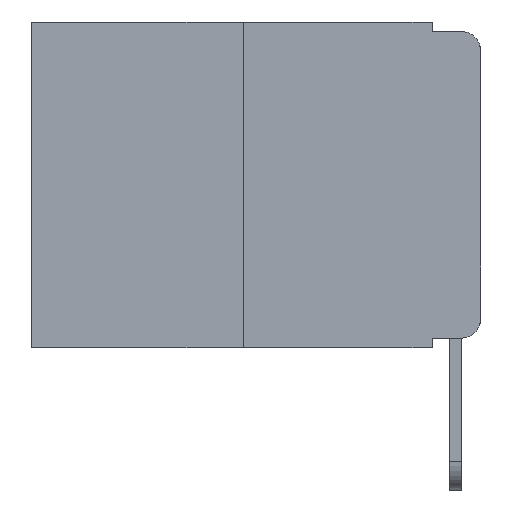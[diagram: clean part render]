
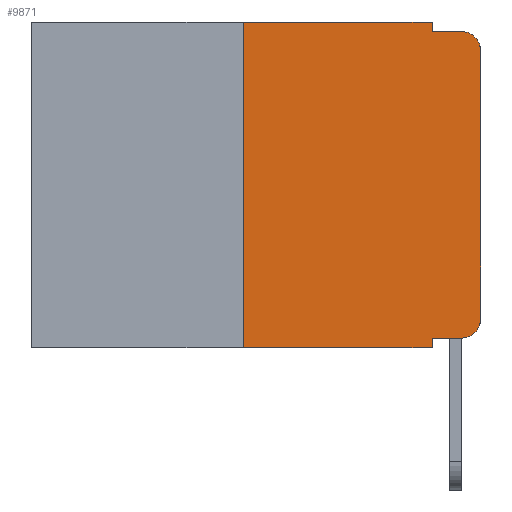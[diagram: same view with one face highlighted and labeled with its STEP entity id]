
A CAD part, left-side view. The second image highlights one B-rep face of the part: STEP entity #9871.
In plain terms, the highlighted planar face has unit normal (-1, 0, 0).
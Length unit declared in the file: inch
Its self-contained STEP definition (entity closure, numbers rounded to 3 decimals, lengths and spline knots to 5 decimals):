
#379 = DIRECTION ( 'NONE',  ( 0., 0., -1. ) ) ;
#418 = VECTOR ( 'NONE', #8810, 39.37008 ) ;
#495 = DIRECTION ( 'NONE',  ( 0., 0., -1. ) ) ;
#585 = ORIENTED_EDGE ( 'NONE', *, *, #9537, .T. ) ;
#765 = CARTESIAN_POINT ( 'NONE',  ( 0., 0.473, 0. ) ) ;
#1775 = CARTESIAN_POINT ( 'NONE',  ( 0., 0.473, 0. ) ) ;
#1841 = EDGE_CURVE ( 'NONE', #3556, #6633, #4339, .T. ) ;
#2386 = AXIS2_PLACEMENT_3D ( 'NONE', #2842, #4954, #379 ) ;
#2530 = VERTEX_POINT ( 'NONE', #12695 ) ;
#2642 = ORIENTED_EDGE ( 'NONE', *, *, #1841, .T. ) ;
#2717 = EDGE_LOOP ( 'NONE', ( #585, #4007, #13675, #11287, #14692, #12070, #2642, #13159, #13503, #4212 ) ) ;
#2809 = VERTEX_POINT ( 'NONE', #5738 ) ;
#2842 = CARTESIAN_POINT ( 'NONE',  ( 0., 0.02, -0.313 ) ) ;
#3222 = VERTEX_POINT ( 'NONE', #5618 ) ;
#3536 = DIRECTION ( 'NONE',  ( 0., -1., 0. ) ) ;
#3556 = VERTEX_POINT ( 'NONE', #5832 ) ;
#3585 = VECTOR ( 'NONE', #3536, 39.37008 ) ;
#3656 = VECTOR ( 'NONE', #9471, 39.37008 ) ;
#4007 = ORIENTED_EDGE ( 'NONE', *, *, #11040, .T. ) ;
#4096 = CARTESIAN_POINT ( 'NONE',  ( 0., 0., -0.03 ) ) ;
#4164 = LINE ( 'NONE', #7199, #13109 ) ;
#4197 = EDGE_CURVE ( 'NONE', #3222, #6633, #5877, .T. ) ;
#4212 = ORIENTED_EDGE ( 'NONE', *, *, #8658, .T. ) ;
#4235 = VERTEX_POINT ( 'NONE', #12694 ) ;
#4339 = LINE ( 'NONE', #8033, #3585 ) ;
#4785 = CARTESIAN_POINT ( 'NONE',  ( 0., 0.051, 0. ) ) ;
#4954 = DIRECTION ( 'NONE',  ( -1., 0., 0. ) ) ;
#5037 = LINE ( 'NONE', #11932, #14226 ) ;
#5238 = VECTOR ( 'NONE', #8023, 39.37008 ) ;
#5289 = CARTESIAN_POINT ( 'NONE',  ( 0., 0.051, 0. ) ) ;
#5618 = CARTESIAN_POINT ( 'NONE',  ( 0., 0.051, -0.333 ) ) ;
#5738 = CARTESIAN_POINT ( 'NONE',  ( 0., 0.051, 0. ) ) ;
#5832 = CARTESIAN_POINT ( 'NONE',  ( 0., 0.25, -0.343 ) ) ;
#5877 = LINE ( 'NONE', #4785, #11967 ) ;
#5885 = EDGE_CURVE ( 'NONE', #3556, #14198, #10777, .T. ) ;
#6035 = DIRECTION ( 'NONE',  ( -1., 0., 0. ) ) ;
#6120 = VERTEX_POINT ( 'NONE', #12020 ) ;
#6210 = LINE ( 'NONE', #765, #3656 ) ;
#6511 = DIRECTION ( 'NONE',  ( 0., 0., -1. ) ) ;
#6549 = VERTEX_POINT ( 'NONE', #14312 ) ;
#6633 = VERTEX_POINT ( 'NONE', #14507 ) ;
#7199 = CARTESIAN_POINT ( 'NONE',  ( 0., 0.051, -0.333 ) ) ;
#8023 = DIRECTION ( 'NONE',  ( 0., -1., 0. ) ) ;
#8033 = CARTESIAN_POINT ( 'NONE',  ( 0., 0.473, -0.343 ) ) ;
#8064 = DIRECTION ( 'NONE',  ( 0., 0., -1. ) ) ;
#8095 = CARTESIAN_POINT ( 'NONE',  ( 0., 0.25, 0. ) ) ;
#8373 = CARTESIAN_POINT ( 'NONE',  ( 0., 0.25, 0. ) ) ;
#8441 = DIRECTION ( 'NONE',  ( 0., -1., 0. ) ) ;
#8658 = EDGE_CURVE ( 'NONE', #6549, #2530, #8907, .T. ) ;
#8810 = DIRECTION ( 'NONE',  ( 0., 0., 1. ) ) ;
#8907 = CIRCLE ( 'NONE', #2386, 0.02 ) ;
#9219 = LINE ( 'NONE', #5289, #12091 ) ;
#9471 = DIRECTION ( 'NONE',  ( 0., -1., 0. ) ) ;
#9537 = EDGE_CURVE ( 'NONE', #2530, #12970, #5037, .T. ) ;
#9871 = ADVANCED_FACE ( 'NONE', ( #11884 ), #13983, .F. ) ;
#10777 = LINE ( 'NONE', #8373, #418 ) ;
#10981 = AXIS2_PLACEMENT_3D ( 'NONE', #1775, #15068, #8064 ) ;
#11040 = EDGE_CURVE ( 'NONE', #12970, #4235, #14434, .T. ) ;
#11287 = ORIENTED_EDGE ( 'NONE', *, *, #12400, .F. ) ;
#11884 = FACE_OUTER_BOUND ( 'NONE', #2717, .T. ) ;
#11932 = CARTESIAN_POINT ( 'NONE',  ( 0., 0., 0. ) ) ;
#11967 = VECTOR ( 'NONE', #495, 39.37008 ) ;
#12020 = CARTESIAN_POINT ( 'NONE',  ( 0., 0.051, -0.01 ) ) ;
#12070 = ORIENTED_EDGE ( 'NONE', *, *, #5885, .F. ) ;
#12079 = EDGE_CURVE ( 'NONE', #6120, #4235, #14721, .T. ) ;
#12091 = VECTOR ( 'NONE', #6511, 39.37008 ) ;
#12220 = EDGE_CURVE ( 'NONE', #14198, #2809, #6210, .T. ) ;
#12400 = EDGE_CURVE ( 'NONE', #2809, #6120, #9219, .T. ) ;
#12694 = CARTESIAN_POINT ( 'NONE',  ( 0., 0.02, -0.01 ) ) ;
#12695 = CARTESIAN_POINT ( 'NONE',  ( 0., 0., -0.313 ) ) ;
#12970 = VERTEX_POINT ( 'NONE', #4096 ) ;
#13109 = VECTOR ( 'NONE', #8441, 39.37008 ) ;
#13159 = ORIENTED_EDGE ( 'NONE', *, *, #4197, .F. ) ;
#13247 = CARTESIAN_POINT ( 'NONE',  ( 0., 0.02, -0.03 ) ) ;
#13453 = EDGE_CURVE ( 'NONE', #3222, #6549, #4164, .T. ) ;
#13503 = ORIENTED_EDGE ( 'NONE', *, *, #13453, .T. ) ;
#13675 = ORIENTED_EDGE ( 'NONE', *, *, #12079, .F. ) ;
#13951 = CARTESIAN_POINT ( 'NONE',  ( 0., 0.051, -0.01 ) ) ;
#13983 = PLANE ( 'NONE',  #10981 ) ;
#14198 = VERTEX_POINT ( 'NONE', #8095 ) ;
#14226 = VECTOR ( 'NONE', #15264, 39.37008 ) ;
#14312 = CARTESIAN_POINT ( 'NONE',  ( 0., 0.02, -0.333 ) ) ;
#14366 = DIRECTION ( 'NONE',  ( 0., 0., -1. ) ) ;
#14434 = CIRCLE ( 'NONE', #14648, 0.02 ) ;
#14507 = CARTESIAN_POINT ( 'NONE',  ( 0., 0.051, -0.343 ) ) ;
#14648 = AXIS2_PLACEMENT_3D ( 'NONE', #13247, #6035, #14366 ) ;
#14692 = ORIENTED_EDGE ( 'NONE', *, *, #12220, .F. ) ;
#14721 = LINE ( 'NONE', #13951, #5238 ) ;
#15068 = DIRECTION ( 'NONE',  ( 1., 0., 0. ) ) ;
#15264 = DIRECTION ( 'NONE',  ( 0., 0., 1. ) ) ;
